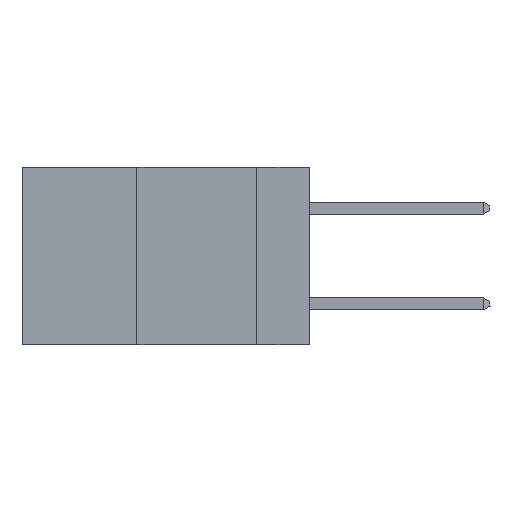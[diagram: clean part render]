
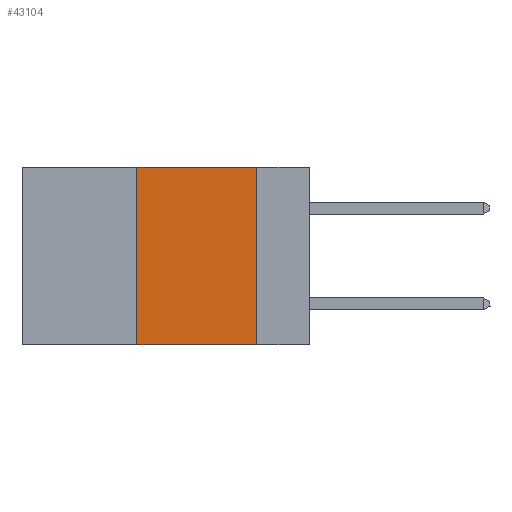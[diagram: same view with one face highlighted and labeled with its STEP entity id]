
A CAD part, left-side view. The second image highlights one B-rep face of the part: STEP entity #43104.
In plain terms, the highlighted planar face has unit normal (-1, 0, 0).
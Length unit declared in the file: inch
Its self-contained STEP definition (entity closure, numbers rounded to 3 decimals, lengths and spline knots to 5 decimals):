
#847 = LINE ( 'NONE', #4555, #17964 ) ;
#2372 = DIRECTION ( 'NONE',  ( 1., 0., 0. ) ) ;
#2650 = VECTOR ( 'NONE', #30073, 39.37008 ) ;
#3388 = ORIENTED_EDGE ( 'NONE', *, *, #5283, .T. ) ;
#4555 = CARTESIAN_POINT ( 'NONE',  ( 0., 0.11, 0. ) ) ;
#5263 = AXIS2_PLACEMENT_3D ( 'NONE', #9610, #2372, #16561 ) ;
#5283 = EDGE_CURVE ( 'NONE', #20857, #18316, #12009, .T. ) ;
#5369 = DIRECTION ( 'NONE',  ( 0., 0., 1. ) ) ;
#7536 = CARTESIAN_POINT ( 'NONE',  ( 0., 0.11, 0. ) ) ;
#9610 = CARTESIAN_POINT ( 'NONE',  ( 0., 0.6, 0. ) ) ;
#12009 = LINE ( 'NONE', #41186, #2650 ) ;
#14366 = EDGE_LOOP ( 'NONE', ( #23423, #24740, #31492, #3388 ) ) ;
#14472 = CARTESIAN_POINT ( 'NONE',  ( 0., 0.36, 0. ) ) ;
#16561 = DIRECTION ( 'NONE',  ( 0., 0., -1. ) ) ;
#17964 = VECTOR ( 'NONE', #28970, 39.37008 ) ;
#18316 = VERTEX_POINT ( 'NONE', #27065 ) ;
#20857 = VERTEX_POINT ( 'NONE', #40938 ) ;
#23423 = ORIENTED_EDGE ( 'NONE', *, *, #29340, .F. ) ;
#24740 = ORIENTED_EDGE ( 'NONE', *, *, #26730, .F. ) ;
#26031 = VERTEX_POINT ( 'NONE', #7536 ) ;
#26256 = VECTOR ( 'NONE', #29944, 39.37008 ) ;
#26382 = CARTESIAN_POINT ( 'NONE',  ( 0., 0.6, 0. ) ) ;
#26730 = EDGE_CURVE ( 'NONE', #27286, #26031, #37987, .T. ) ;
#27065 = CARTESIAN_POINT ( 'NONE',  ( 0., 0.11, -0.37 ) ) ;
#27286 = VERTEX_POINT ( 'NONE', #14472 ) ;
#28970 = DIRECTION ( 'NONE',  ( 0., 0., -1. ) ) ;
#29340 = EDGE_CURVE ( 'NONE', #26031, #18316, #847, .T. ) ;
#29944 = DIRECTION ( 'NONE',  ( 0., -1., 0. ) ) ;
#30073 = DIRECTION ( 'NONE',  ( 0., -1., 0. ) ) ;
#31492 = ORIENTED_EDGE ( 'NONE', *, *, #35170, .F. ) ;
#33591 = VECTOR ( 'NONE', #5369, 39.37008 ) ;
#35170 = EDGE_CURVE ( 'NONE', #20857, #27286, #43144, .T. ) ;
#37987 = LINE ( 'NONE', #26382, #26256 ) ;
#40888 = CARTESIAN_POINT ( 'NONE',  ( 0., 0.36, 0. ) ) ;
#40938 = CARTESIAN_POINT ( 'NONE',  ( 0., 0.36, -0.37 ) ) ;
#41186 = CARTESIAN_POINT ( 'NONE',  ( 0., 0.6, -0.37 ) ) ;
#43104 = ADVANCED_FACE ( 'NONE', ( #45933 ), #45355, .F. ) ;
#43144 = LINE ( 'NONE', #40888, #33591 ) ;
#45355 = PLANE ( 'NONE',  #5263 ) ;
#45933 = FACE_OUTER_BOUND ( 'NONE', #14366, .T. ) ;
